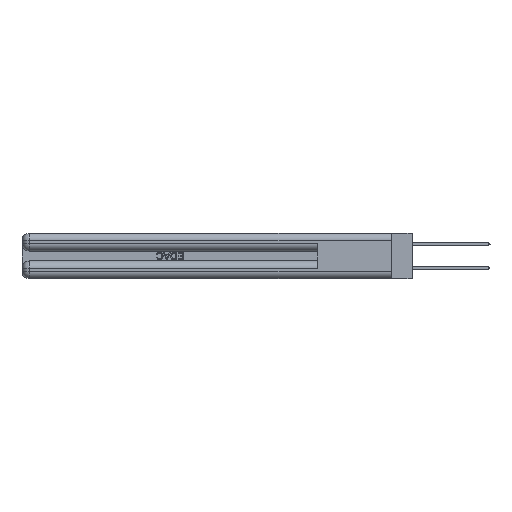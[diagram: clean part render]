
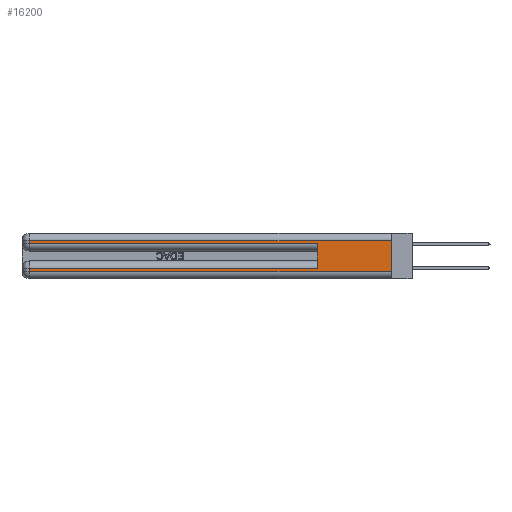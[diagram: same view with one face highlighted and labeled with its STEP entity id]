
A CAD part, left-side view. The second image highlights one B-rep face of the part: STEP entity #16200.
In plain terms, the highlighted planar face has unit normal (-1, 0, 0).
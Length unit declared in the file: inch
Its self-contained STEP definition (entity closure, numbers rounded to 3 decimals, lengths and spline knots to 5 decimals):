
#191 = CARTESIAN_POINT ( 'NONE',  ( 0., 2.94, 0.37 ) ) ;
#244 = LINE ( 'NONE', #37854, #39216 ) ;
#535 = EDGE_CURVE ( 'NONE', #5095, #36448, #22907, .T. ) ;
#813 = CARTESIAN_POINT ( 'NONE',  ( 0., 0., 0.37 ) ) ;
#973 = DIRECTION ( 'NONE',  ( 1., 0., 0. ) ) ;
#3096 = DIRECTION ( 'NONE',  ( 0., 0., -1. ) ) ;
#3470 = VECTOR ( 'NONE', #42199, 39.37008 ) ;
#4352 = DIRECTION ( 'NONE',  ( 0., 0., -1. ) ) ;
#5095 = VERTEX_POINT ( 'NONE', #45328 ) ;
#5181 = EDGE_LOOP ( 'NONE', ( #29561, #19978, #21778, #26502, #14377, #45203, #32178, #42311 ) ) ;
#5625 = DIRECTION ( 'NONE',  ( 0., -1., 0. ) ) ;
#6134 = EDGE_CURVE ( 'NONE', #7438, #29793, #25892, .T. ) ;
#6698 = CARTESIAN_POINT ( 'NONE',  ( 0., 2.94, 0.37 ) ) ;
#6938 = VECTOR ( 'NONE', #3096, 39.37008 ) ;
#7438 = VERTEX_POINT ( 'NONE', #12240 ) ;
#8399 = DIRECTION ( 'NONE',  ( 0., 1., 0. ) ) ;
#10272 = EDGE_CURVE ( 'NONE', #36448, #44612, #21253, .T. ) ;
#10490 = DIRECTION ( 'NONE',  ( 0., -1., 0. ) ) ;
#10598 = CARTESIAN_POINT ( 'NONE',  ( 0., 0., 0.37 ) ) ;
#12240 = CARTESIAN_POINT ( 'NONE',  ( 0., 0., 0.31 ) ) ;
#13346 = CARTESIAN_POINT ( 'NONE',  ( 0., 0., 0.06 ) ) ;
#13477 = EDGE_CURVE ( 'NONE', #36299, #44656, #244, .T. ) ;
#14129 = CARTESIAN_POINT ( 'NONE',  ( 0., 0.6, 0.285 ) ) ;
#14377 = ORIENTED_EDGE ( 'NONE', *, *, #13477, .F. ) ;
#16200 = ADVANCED_FACE ( 'NONE', ( #21781 ), #19297, .F. ) ;
#16728 = EDGE_CURVE ( 'NONE', #23232, #44656, #25694, .T. ) ;
#18810 = CARTESIAN_POINT ( 'NONE',  ( 0., 2.94, 0.06 ) ) ;
#19038 = VECTOR ( 'NONE', #42057, 39.37008 ) ;
#19297 = PLANE ( 'NONE',  #32584 ) ;
#19978 = ORIENTED_EDGE ( 'NONE', *, *, #6134, .T. ) ;
#21253 = LINE ( 'NONE', #13346, #29745 ) ;
#21436 = CARTESIAN_POINT ( 'NONE',  ( 0., 0., 0.06 ) ) ;
#21778 = ORIENTED_EDGE ( 'NONE', *, *, #27335, .T. ) ;
#21781 = FACE_OUTER_BOUND ( 'NONE', #5181, .T. ) ;
#22907 = LINE ( 'NONE', #6698, #3470 ) ;
#23232 = VERTEX_POINT ( 'NONE', #41482 ) ;
#23827 = VECTOR ( 'NONE', #8399, 39.37008 ) ;
#24421 = CARTESIAN_POINT ( 'NONE',  ( 0., 2.94, 0.31 ) ) ;
#25694 = LINE ( 'NONE', #31143, #27441 ) ;
#25892 = LINE ( 'NONE', #45235, #19038 ) ;
#26489 = DIRECTION ( 'NONE',  ( 0., 0., -1. ) ) ;
#26502 = ORIENTED_EDGE ( 'NONE', *, *, #16728, .T. ) ;
#27335 = EDGE_CURVE ( 'NONE', #29793, #23232, #35360, .T. ) ;
#27441 = VECTOR ( 'NONE', #10490, 39.37008 ) ;
#27764 = EDGE_CURVE ( 'NONE', #36299, #5095, #35259, .T. ) ;
#29561 = ORIENTED_EDGE ( 'NONE', *, *, #41090, .F. ) ;
#29745 = VECTOR ( 'NONE', #5625, 39.37008 ) ;
#29793 = VERTEX_POINT ( 'NONE', #24421 ) ;
#31143 = CARTESIAN_POINT ( 'NONE',  ( 0., 0., 0.285 ) ) ;
#32178 = ORIENTED_EDGE ( 'NONE', *, *, #535, .T. ) ;
#32584 = AXIS2_PLACEMENT_3D ( 'NONE', #813, #973, #26489 ) ;
#35259 = LINE ( 'NONE', #44998, #23827 ) ;
#35360 = LINE ( 'NONE', #191, #46797 ) ;
#36299 = VERTEX_POINT ( 'NONE', #36409 ) ;
#36409 = CARTESIAN_POINT ( 'NONE',  ( 0., 0.6, 0.085 ) ) ;
#36448 = VERTEX_POINT ( 'NONE', #18810 ) ;
#36625 = LINE ( 'NONE', #10598, #6938 ) ;
#37854 = CARTESIAN_POINT ( 'NONE',  ( 0., 0.6, 0.145 ) ) ;
#39216 = VECTOR ( 'NONE', #41548, 39.37008 ) ;
#41090 = EDGE_CURVE ( 'NONE', #7438, #44612, #36625, .T. ) ;
#41482 = CARTESIAN_POINT ( 'NONE',  ( 0., 2.94, 0.285 ) ) ;
#41548 = DIRECTION ( 'NONE',  ( 0., 0., 1. ) ) ;
#42057 = DIRECTION ( 'NONE',  ( 0., 1., 0. ) ) ;
#42199 = DIRECTION ( 'NONE',  ( 0., 0., -1. ) ) ;
#42311 = ORIENTED_EDGE ( 'NONE', *, *, #10272, .T. ) ;
#44612 = VERTEX_POINT ( 'NONE', #21436 ) ;
#44656 = VERTEX_POINT ( 'NONE', #14129 ) ;
#44998 = CARTESIAN_POINT ( 'NONE',  ( 0., 0., 0.085 ) ) ;
#45203 = ORIENTED_EDGE ( 'NONE', *, *, #27764, .T. ) ;
#45235 = CARTESIAN_POINT ( 'NONE',  ( 0., 0., 0.31 ) ) ;
#45328 = CARTESIAN_POINT ( 'NONE',  ( 0., 2.94, 0.085 ) ) ;
#46797 = VECTOR ( 'NONE', #4352, 39.37008 ) ;
